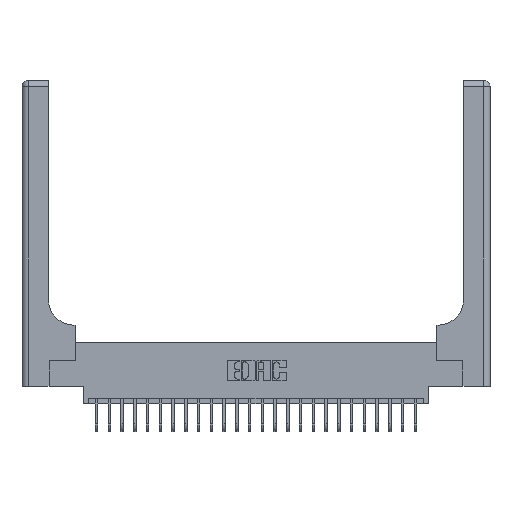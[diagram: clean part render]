
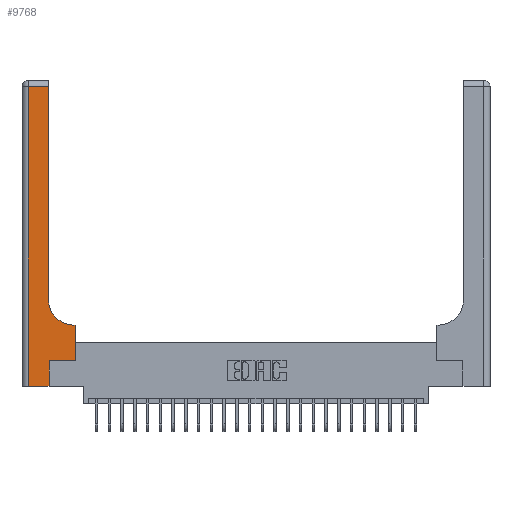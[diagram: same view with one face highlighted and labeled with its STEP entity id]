
A CAD part, top view. The second image highlights one B-rep face of the part: STEP entity #9768.
In plain terms, the highlighted planar face has unit normal (0, 0, 1).
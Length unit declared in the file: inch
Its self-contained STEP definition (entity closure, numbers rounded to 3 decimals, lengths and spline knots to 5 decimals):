
#53 = EDGE_CURVE ( 'NONE', #12339, #10008, #1754, .T. ) ;
#106 = DIRECTION ( 'NONE',  ( 1., 0., 0. ) ) ;
#191 = CARTESIAN_POINT ( 'NONE',  ( 0., 0., 0.37 ) ) ;
#366 = CARTESIAN_POINT ( 'NONE',  ( 0.528, 0.6, 0.37 ) ) ;
#602 = CARTESIAN_POINT ( 'NONE',  ( 0.265, 0., 0.37 ) ) ;
#971 = CARTESIAN_POINT ( 'NONE',  ( 0.265, 0., 0.37 ) ) ;
#1026 = VECTOR ( 'NONE', #21005, 39.37008 ) ;
#1161 = CARTESIAN_POINT ( 'NONE',  ( 0.528, 0.25, 0.37 ) ) ;
#1169 = VECTOR ( 'NONE', #10881, 39.37008 ) ;
#1534 = CARTESIAN_POINT ( 'NONE',  ( 0., 3., 0.37 ) ) ;
#1754 = LINE ( 'NONE', #8498, #20605 ) ;
#2031 = LINE ( 'NONE', #4773, #11717 ) ;
#2383 = CARTESIAN_POINT ( 'NONE',  ( 0.26, 3., 0.37 ) ) ;
#3258 = ORIENTED_EDGE ( 'NONE', *, *, #13155, .T. ) ;
#3401 = PLANE ( 'NONE',  #22363 ) ;
#4249 = VERTEX_POINT ( 'NONE', #14535 ) ;
#4392 = ORIENTED_EDGE ( 'NONE', *, *, #53, .T. ) ;
#4597 = ORIENTED_EDGE ( 'NONE', *, *, #10647, .T. ) ;
#4773 = CARTESIAN_POINT ( 'NONE',  ( 0., 2.94, 0.37 ) ) ;
#5210 = DIRECTION ( 'NONE',  ( 0., 0., -1. ) ) ;
#6571 = EDGE_CURVE ( 'NONE', #14095, #20309, #2031, .T. ) ;
#6698 = CARTESIAN_POINT ( 'NONE',  ( 0.51, 0.85, 0.37 ) ) ;
#6726 = VECTOR ( 'NONE', #19563, 39.37008 ) ;
#7336 = VECTOR ( 'NONE', #106, 39.37008 ) ;
#7473 = CARTESIAN_POINT ( 'NONE',  ( 0.26, 2.94, 0.37 ) ) ;
#8498 = CARTESIAN_POINT ( 'NONE',  ( 0.26, 0.6, 0.37 ) ) ;
#8541 = DIRECTION ( 'NONE',  ( 1., 0., 0. ) ) ;
#8554 = CARTESIAN_POINT ( 'NONE',  ( 0.265, 0.25, 0.37 ) ) ;
#8577 = DIRECTION ( 'NONE',  ( -1., 0., 0. ) ) ;
#9242 = ORIENTED_EDGE ( 'NONE', *, *, #17575, .T. ) ;
#9350 = VERTEX_POINT ( 'NONE', #12886 ) ;
#9419 = VECTOR ( 'NONE', #15751, 39.37008 ) ;
#9768 = ADVANCED_FACE ( 'NONE', ( #21447 ), #3401, .F. ) ;
#9924 = VERTEX_POINT ( 'NONE', #14907 ) ;
#10008 = VERTEX_POINT ( 'NONE', #22394 ) ;
#10157 = LINE ( 'NONE', #971, #1026 ) ;
#10579 = ORIENTED_EDGE ( 'NONE', *, *, #6571, .T. ) ;
#10647 = EDGE_CURVE ( 'NONE', #10903, #14095, #14517, .T. ) ;
#10669 = CARTESIAN_POINT ( 'NONE',  ( 0.06, 2.94, 0.37 ) ) ;
#10881 = DIRECTION ( 'NONE',  ( 0., -1., 0. ) ) ;
#10903 = VERTEX_POINT ( 'NONE', #17423 ) ;
#11459 = DIRECTION ( 'NONE',  ( 0., 1., 0. ) ) ;
#11565 = LINE ( 'NONE', #8554, #6726 ) ;
#11717 = VECTOR ( 'NONE', #17537, 39.37008 ) ;
#12339 = VERTEX_POINT ( 'NONE', #366 ) ;
#12886 = CARTESIAN_POINT ( 'NONE',  ( 0.265, 0.25, 0.37 ) ) ;
#12944 = ORIENTED_EDGE ( 'NONE', *, *, #13290, .T. ) ;
#12962 = CIRCLE ( 'NONE', #21216, 0.25 ) ;
#13155 = EDGE_CURVE ( 'NONE', #20658, #9350, #10157, .T. ) ;
#13290 = EDGE_CURVE ( 'NONE', #9350, #4249, #11565, .T. ) ;
#13374 = VECTOR ( 'NONE', #11459, 39.37008 ) ;
#14095 = VERTEX_POINT ( 'NONE', #7473 ) ;
#14517 = LINE ( 'NONE', #2383, #13374 ) ;
#14535 = CARTESIAN_POINT ( 'NONE',  ( 0.528, 0.25, 0.37 ) ) ;
#14907 = CARTESIAN_POINT ( 'NONE',  ( 0.06, 0., 0.37 ) ) ;
#15004 = EDGE_LOOP ( 'NONE', ( #4597, #10579, #20296, #22120, #3258, #12944, #18386, #4392, #9242 ) ) ;
#15751 = DIRECTION ( 'NONE',  ( 0., 1., 0. ) ) ;
#15946 = EDGE_CURVE ( 'NONE', #9924, #20658, #21919, .T. ) ;
#17423 = CARTESIAN_POINT ( 'NONE',  ( 0.26, 0.85, 0.37 ) ) ;
#17537 = DIRECTION ( 'NONE',  ( -1., 0., 0. ) ) ;
#17575 = EDGE_CURVE ( 'NONE', #10008, #10903, #12962, .T. ) ;
#17994 = DIRECTION ( 'NONE',  ( -1., 0., 0. ) ) ;
#18386 = ORIENTED_EDGE ( 'NONE', *, *, #20730, .T. ) ;
#19257 = EDGE_CURVE ( 'NONE', #20309, #9924, #21176, .T. ) ;
#19473 = DIRECTION ( 'NONE',  ( 0., 0., -1. ) ) ;
#19563 = DIRECTION ( 'NONE',  ( 1., 0., 0. ) ) ;
#20279 = LINE ( 'NONE', #1161, #9419 ) ;
#20296 = ORIENTED_EDGE ( 'NONE', *, *, #19257, .T. ) ;
#20309 = VERTEX_POINT ( 'NONE', #10669 ) ;
#20605 = VECTOR ( 'NONE', #8577, 39.37008 ) ;
#20658 = VERTEX_POINT ( 'NONE', #602 ) ;
#20730 = EDGE_CURVE ( 'NONE', #4249, #12339, #20279, .T. ) ;
#21005 = DIRECTION ( 'NONE',  ( 0., 1., 0. ) ) ;
#21176 = LINE ( 'NONE', #23685, #1169 ) ;
#21216 = AXIS2_PLACEMENT_3D ( 'NONE', #6698, #19473, #8541 ) ;
#21447 = FACE_OUTER_BOUND ( 'NONE', #15004, .T. ) ;
#21919 = LINE ( 'NONE', #191, #7336 ) ;
#22120 = ORIENTED_EDGE ( 'NONE', *, *, #15946, .T. ) ;
#22363 = AXIS2_PLACEMENT_3D ( 'NONE', #1534, #5210, #17994 ) ;
#22394 = CARTESIAN_POINT ( 'NONE',  ( 0.51, 0.6, 0.37 ) ) ;
#23685 = CARTESIAN_POINT ( 'NONE',  ( 0.06, 3., 0.37 ) ) ;
